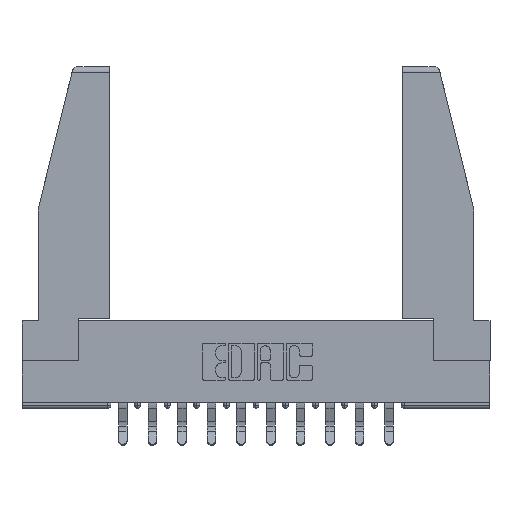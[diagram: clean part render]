
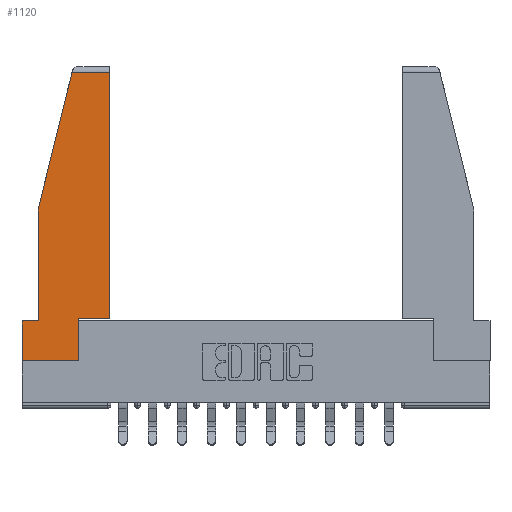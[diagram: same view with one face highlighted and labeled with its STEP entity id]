
A CAD part, top view. The second image highlights one B-rep face of the part: STEP entity #1120.
In plain terms, the highlighted planar face has unit normal (0, 0, 1).
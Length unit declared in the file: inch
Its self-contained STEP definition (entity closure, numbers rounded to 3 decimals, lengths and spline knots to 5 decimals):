
#61 = CARTESIAN_POINT ( 'NONE',  ( 0., 0.21, 0. ) ) ;
#186 = LINE ( 'NONE', #10630, #17014 ) ;
#231 = DIRECTION ( 'NONE',  ( -1., 0., 0. ) ) ;
#310 = EDGE_CURVE ( 'NONE', #5617, #647, #16061, .T. ) ;
#380 = DIRECTION ( 'NONE',  ( -1., 0., 0. ) ) ;
#516 = VECTOR ( 'NONE', #231, 39.37008 ) ;
#647 = VERTEX_POINT ( 'NONE', #13204 ) ;
#776 = CARTESIAN_POINT ( 'NONE',  ( 0., 0.21, 0. ) ) ;
#1120 = ADVANCED_FACE ( 'NONE', ( #11425 ), #16422, .T. ) ;
#1186 = VERTEX_POINT ( 'NONE', #13792 ) ;
#1569 = ORIENTED_EDGE ( 'NONE', *, *, #310, .T. ) ;
#1606 = CARTESIAN_POINT ( 'NONE',  ( 0., 1.52, 0. ) ) ;
#2140 = EDGE_CURVE ( 'NONE', #4204, #17170, #5851, .T. ) ;
#2304 = VECTOR ( 'NONE', #9476, 39.37008 ) ;
#2713 = CARTESIAN_POINT ( 'NONE',  ( 0.086, 0.8, 0. ) ) ;
#2882 = ORIENTED_EDGE ( 'NONE', *, *, #16198, .T. ) ;
#3190 = DIRECTION ( 'NONE',  ( 1., 0., 0. ) ) ;
#3217 = CARTESIAN_POINT ( 'NONE',  ( 0., 0., 0. ) ) ;
#3409 = DIRECTION ( 'NONE',  ( 0., -1., 0. ) ) ;
#3532 = EDGE_CURVE ( 'NONE', #647, #7225, #8266, .T. ) ;
#3871 = ORIENTED_EDGE ( 'NONE', *, *, #8607, .T. ) ;
#4009 = CARTESIAN_POINT ( 'NONE',  ( 0.297, 0.223, 0. ) ) ;
#4204 = VERTEX_POINT ( 'NONE', #4899 ) ;
#4272 = ORIENTED_EDGE ( 'NONE', *, *, #2140, .T. ) ;
#4643 = ORIENTED_EDGE ( 'NONE', *, *, #3532, .T. ) ;
#4815 = DIRECTION ( 'NONE',  ( 1., 0., 0. ) ) ;
#4860 = CARTESIAN_POINT ( 'NONE',  ( 0.086, 0.21, 0. ) ) ;
#4899 = CARTESIAN_POINT ( 'NONE',  ( 0.461, 0.223, 0. ) ) ;
#5070 = VERTEX_POINT ( 'NONE', #17099 ) ;
#5309 = VECTOR ( 'NONE', #3409, 39.37008 ) ;
#5411 = DIRECTION ( 'NONE',  ( 0., 0., 1. ) ) ;
#5617 = VERTEX_POINT ( 'NONE', #4860 ) ;
#5851 = LINE ( 'NONE', #9663, #2304 ) ;
#5998 = VERTEX_POINT ( 'NONE', #4009 ) ;
#6746 = AXIS2_PLACEMENT_3D ( 'NONE', #15837, #5411, #9433 ) ;
#6758 = DIRECTION ( 'NONE',  ( 0., 1., 0. ) ) ;
#6876 = EDGE_CURVE ( 'NONE', #1186, #11297, #15346, .T. ) ;
#6955 = EDGE_CURVE ( 'NONE', #5070, #5998, #186, .T. ) ;
#7225 = VERTEX_POINT ( 'NONE', #3217 ) ;
#7227 = ORIENTED_EDGE ( 'NONE', *, *, #16366, .T. ) ;
#7460 = ORIENTED_EDGE ( 'NONE', *, *, #6955, .T. ) ;
#7540 = CARTESIAN_POINT ( 'NONE',  ( 0.461, 1.52, 0. ) ) ;
#8266 = LINE ( 'NONE', #776, #5309 ) ;
#8421 = VECTOR ( 'NONE', #15200, 39.37008 ) ;
#8607 = EDGE_CURVE ( 'NONE', #17170, #1186, #14623, .T. ) ;
#9066 = CARTESIAN_POINT ( 'NONE',  ( 0.086, 0.8, 0. ) ) ;
#9285 = ORIENTED_EDGE ( 'NONE', *, *, #6876, .T. ) ;
#9433 = DIRECTION ( 'NONE',  ( 1., 0., 0. ) ) ;
#9476 = DIRECTION ( 'NONE',  ( 0., 1., 0. ) ) ;
#9663 = CARTESIAN_POINT ( 'NONE',  ( 0.461, 0.223, 0. ) ) ;
#10287 = EDGE_CURVE ( 'NONE', #11297, #5617, #12862, .T. ) ;
#10630 = CARTESIAN_POINT ( 'NONE',  ( 0.297, 0., 0. ) ) ;
#10681 = EDGE_LOOP ( 'NONE', ( #4272, #3871, #9285, #17222, #1569, #4643, #2882, #7460, #7227 ) ) ;
#11271 = CARTESIAN_POINT ( 'NONE',  ( 0.297, 0.223, 0. ) ) ;
#11297 = VERTEX_POINT ( 'NONE', #9066 ) ;
#11425 = FACE_OUTER_BOUND ( 'NONE', #10681, .T. ) ;
#11742 = VECTOR ( 'NONE', #17166, 39.37008 ) ;
#12862 = LINE ( 'NONE', #2713, #8421 ) ;
#13204 = CARTESIAN_POINT ( 'NONE',  ( 0., 0.21, 0. ) ) ;
#13652 = VECTOR ( 'NONE', #4815, 39.37008 ) ;
#13792 = CARTESIAN_POINT ( 'NONE',  ( 0.2636, 1.52, 0. ) ) ;
#14062 = VECTOR ( 'NONE', #3190, 39.37008 ) ;
#14077 = LINE ( 'NONE', #15718, #13652 ) ;
#14456 = LINE ( 'NONE', #11271, #14062 ) ;
#14623 = LINE ( 'NONE', #1606, #16943 ) ;
#15200 = DIRECTION ( 'NONE',  ( 0., -1., 0. ) ) ;
#15346 = LINE ( 'NONE', #17049, #11742 ) ;
#15718 = CARTESIAN_POINT ( 'NONE',  ( 0., 0., 0. ) ) ;
#15837 = CARTESIAN_POINT ( 'NONE',  ( 0., 0., 0. ) ) ;
#16061 = LINE ( 'NONE', #61, #516 ) ;
#16198 = EDGE_CURVE ( 'NONE', #7225, #5070, #14077, .T. ) ;
#16366 = EDGE_CURVE ( 'NONE', #5998, #4204, #14456, .T. ) ;
#16422 = PLANE ( 'NONE',  #6746 ) ;
#16943 = VECTOR ( 'NONE', #380, 39.37008 ) ;
#17014 = VECTOR ( 'NONE', #6758, 39.37008 ) ;
#17049 = CARTESIAN_POINT ( 'NONE',  ( 0.271, 1.55, 0. ) ) ;
#17099 = CARTESIAN_POINT ( 'NONE',  ( 0.297, 0., 0. ) ) ;
#17166 = DIRECTION ( 'NONE',  ( -0.239, -0.971, 0. ) ) ;
#17170 = VERTEX_POINT ( 'NONE', #7540 ) ;
#17222 = ORIENTED_EDGE ( 'NONE', *, *, #10287, .T. ) ;
